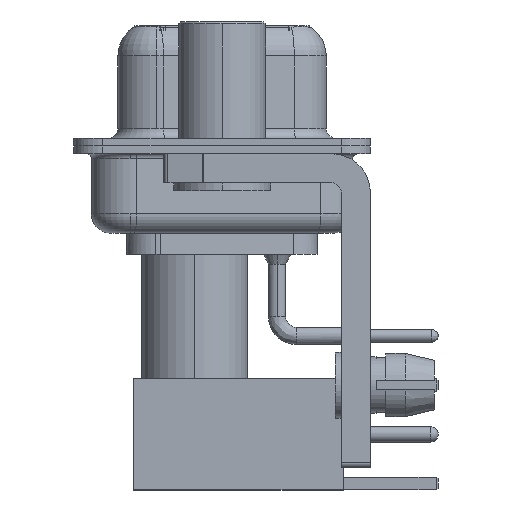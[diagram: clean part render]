
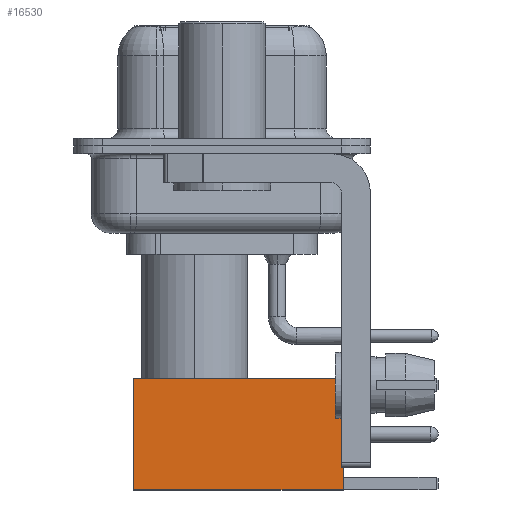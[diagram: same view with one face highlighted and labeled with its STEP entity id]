
A CAD part, left-side view. The second image highlights one B-rep face of the part: STEP entity #16530.
In plain terms, the highlighted face is planar.
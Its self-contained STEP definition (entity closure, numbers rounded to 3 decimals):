
#846 = CARTESIAN_POINT ( 'NONE',  ( 2.875, 2.875, 0. ) ) ;
#1578 = LINE ( 'NONE', #22780, #22031 ) ;
#1823 = LINE ( 'NONE', #5991, #23750 ) ;
#2527 = VECTOR ( 'NONE', #12895, 1000. ) ;
#3064 = EDGE_LOOP ( 'NONE', ( #26903, #6509, #24116, #10789 ) ) ;
#3450 = DIRECTION ( 'NONE',  ( 0., 0., 1. ) ) ;
#3587 = CARTESIAN_POINT ( 'NONE',  ( -2.875, 2.875, 0. ) ) ;
#3685 = AXIS2_PLACEMENT_3D ( 'NONE', #846, #28917, #3450 ) ;
#4340 = VERTEX_POINT ( 'NONE', #20640 ) ;
#5991 = CARTESIAN_POINT ( 'NONE',  ( 0., 2.875, 10.82 ) ) ;
#6334 = VERTEX_POINT ( 'NONE', #12129 ) ;
#6509 = ORIENTED_EDGE ( 'NONE', *, *, #8138, .T. ) ;
#7733 = PLANE ( 'NONE',  #3685 ) ;
#7961 = EDGE_CURVE ( 'NONE', #10944, #6334, #26912, .T. ) ;
#8012 = CARTESIAN_POINT ( 'NONE',  ( 2.875, 2.875, 0. ) ) ;
#8138 = EDGE_CURVE ( 'NONE', #16576, #6334, #1578, .T. ) ;
#10697 = DIRECTION ( 'NONE',  ( -1., 0., 0. ) ) ;
#10789 = ORIENTED_EDGE ( 'NONE', *, *, #18946, .F. ) ;
#10944 = VERTEX_POINT ( 'NONE', #25655 ) ;
#11414 = EDGE_CURVE ( 'NONE', #4340, #16576, #20588, .T. ) ;
#11434 = DIRECTION ( 'NONE',  ( 0., 0., -1. ) ) ;
#12129 = CARTESIAN_POINT ( 'NONE',  ( -2.875, 2.875, 0. ) ) ;
#12895 = DIRECTION ( 'NONE',  ( 0., 0., -1. ) ) ;
#16530 = ADVANCED_FACE ( 'NONE', ( #24043 ), #7733, .T. ) ;
#16576 = VERTEX_POINT ( 'NONE', #20512 ) ;
#18946 = EDGE_CURVE ( 'NONE', #4340, #10944, #1823, .T. ) ;
#20207 = DIRECTION ( 'NONE',  ( -1., 0., 0. ) ) ;
#20512 = CARTESIAN_POINT ( 'NONE',  ( 2.875, 2.875, 0. ) ) ;
#20588 = LINE ( 'NONE', #8012, #22986 ) ;
#20640 = CARTESIAN_POINT ( 'NONE',  ( 2.875, 2.875, 10.82 ) ) ;
#22031 = VECTOR ( 'NONE', #20207, 1000. ) ;
#22780 = CARTESIAN_POINT ( 'NONE',  ( 0., 2.875, 0. ) ) ;
#22986 = VECTOR ( 'NONE', #11434, 1000. ) ;
#23750 = VECTOR ( 'NONE', #10697, 1000. ) ;
#24043 = FACE_OUTER_BOUND ( 'NONE', #3064, .T. ) ;
#24116 = ORIENTED_EDGE ( 'NONE', *, *, #7961, .F. ) ;
#25655 = CARTESIAN_POINT ( 'NONE',  ( -2.875, 2.875, 10.82 ) ) ;
#26903 = ORIENTED_EDGE ( 'NONE', *, *, #11414, .T. ) ;
#26912 = LINE ( 'NONE', #3587, #2527 ) ;
#28917 = DIRECTION ( 'NONE',  ( 0., 1., 0. ) ) ;
